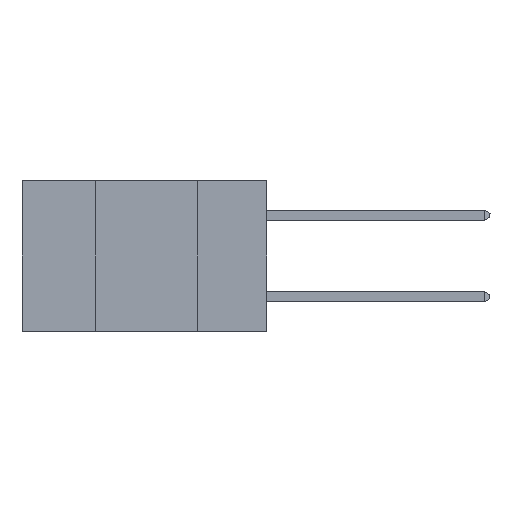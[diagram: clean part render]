
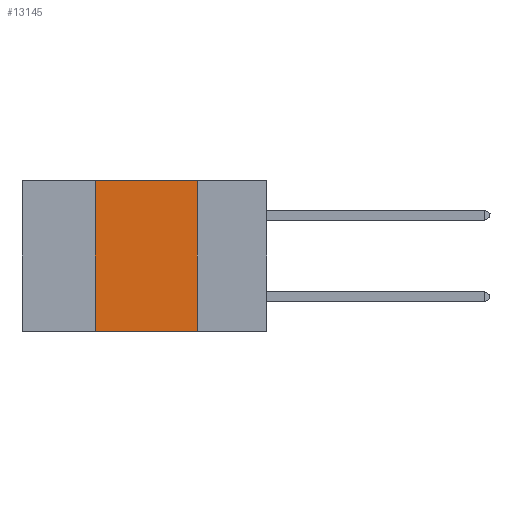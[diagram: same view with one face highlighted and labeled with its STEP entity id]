
A CAD part, left-side view. The second image highlights one B-rep face of the part: STEP entity #13145.
In plain terms, the highlighted planar face has unit normal (-1, 0, 0).
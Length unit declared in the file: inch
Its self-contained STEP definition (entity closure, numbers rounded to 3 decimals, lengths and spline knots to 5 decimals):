
#1499 = CARTESIAN_POINT ( 'NONE',  ( 0., 0.42, 0. ) ) ;
#1754 = VERTEX_POINT ( 'NONE', #3274 ) ;
#1934 = VECTOR ( 'NONE', #17501, 39.37008 ) ;
#2340 = ORIENTED_EDGE ( 'NONE', *, *, #25169, .F. ) ;
#3274 = CARTESIAN_POINT ( 'NONE',  ( 0., 0.17, -0.37 ) ) ;
#3304 = DIRECTION ( 'NONE',  ( 0., 0., -1. ) ) ;
#3350 = CARTESIAN_POINT ( 'NONE',  ( 0., 0.17, 0. ) ) ;
#3952 = VECTOR ( 'NONE', #7095, 39.37008 ) ;
#7095 = DIRECTION ( 'NONE',  ( 0., 0., 1. ) ) ;
#7619 = VERTEX_POINT ( 'NONE', #25003 ) ;
#8227 = CARTESIAN_POINT ( 'NONE',  ( 0., 0.6, 0. ) ) ;
#8441 = AXIS2_PLACEMENT_3D ( 'NONE', #20802, #18495, #3304 ) ;
#8747 = EDGE_CURVE ( 'NONE', #22704, #1754, #21756, .T. ) ;
#9511 = VECTOR ( 'NONE', #15443, 39.37008 ) ;
#11254 = LINE ( 'NONE', #13402, #3952 ) ;
#11916 = CARTESIAN_POINT ( 'NONE',  ( 0., 0.42, -0.37 ) ) ;
#12108 = DIRECTION ( 'NONE',  ( 0., 0., -1. ) ) ;
#13145 = ADVANCED_FACE ( 'NONE', ( #24686 ), #15932, .F. ) ;
#13402 = CARTESIAN_POINT ( 'NONE',  ( 0., 0.42, 0. ) ) ;
#14094 = EDGE_CURVE ( 'NONE', #7619, #1754, #25151, .T. ) ;
#14191 = EDGE_LOOP ( 'NONE', ( #14511, #2340, #28156, #27480 ) ) ;
#14511 = ORIENTED_EDGE ( 'NONE', *, *, #14094, .F. ) ;
#15443 = DIRECTION ( 'NONE',  ( 0., -1., 0. ) ) ;
#15932 = PLANE ( 'NONE',  #8441 ) ;
#17501 = DIRECTION ( 'NONE',  ( 0., -1., 0. ) ) ;
#17766 = EDGE_CURVE ( 'NONE', #22704, #23704, #11254, .T. ) ;
#18495 = DIRECTION ( 'NONE',  ( 1., 0., 0. ) ) ;
#19898 = CARTESIAN_POINT ( 'NONE',  ( 0., 0.6, -0.37 ) ) ;
#20802 = CARTESIAN_POINT ( 'NONE',  ( 0., 0.6, 0. ) ) ;
#21756 = LINE ( 'NONE', #19898, #9511 ) ;
#22643 = VECTOR ( 'NONE', #12108, 39.37008 ) ;
#22704 = VERTEX_POINT ( 'NONE', #11916 ) ;
#23704 = VERTEX_POINT ( 'NONE', #1499 ) ;
#24131 = LINE ( 'NONE', #8227, #1934 ) ;
#24686 = FACE_OUTER_BOUND ( 'NONE', #14191, .T. ) ;
#25003 = CARTESIAN_POINT ( 'NONE',  ( 0., 0.17, 0. ) ) ;
#25151 = LINE ( 'NONE', #3350, #22643 ) ;
#25169 = EDGE_CURVE ( 'NONE', #23704, #7619, #24131, .T. ) ;
#27480 = ORIENTED_EDGE ( 'NONE', *, *, #8747, .T. ) ;
#28156 = ORIENTED_EDGE ( 'NONE', *, *, #17766, .F. ) ;
